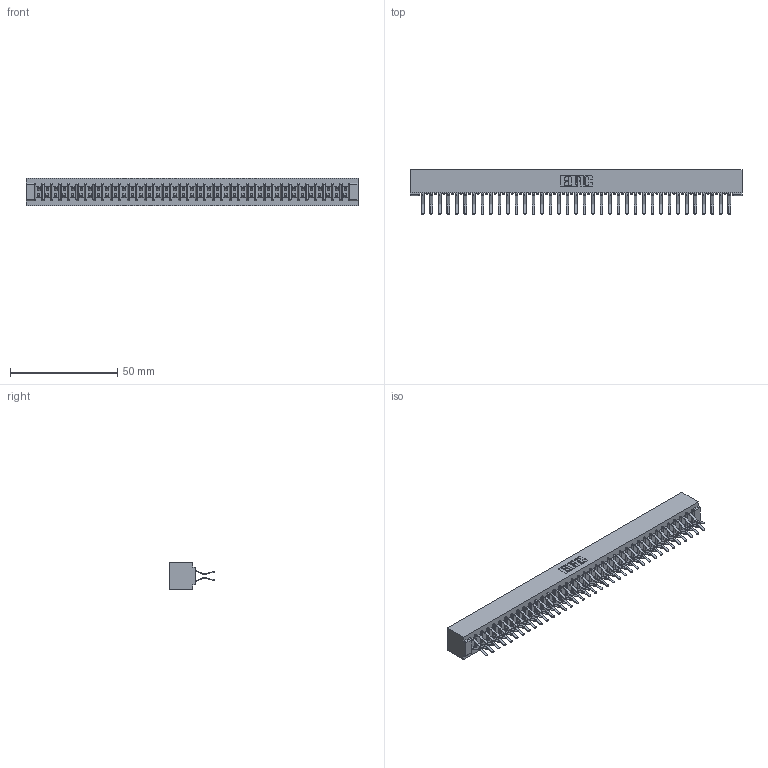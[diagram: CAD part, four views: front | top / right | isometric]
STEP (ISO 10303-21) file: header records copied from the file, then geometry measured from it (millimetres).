
FILE_DESCRIPTION (( 'STEP AP203' ), '1' );
FILE_NAME ('357-074-560-201.STEP', '2018-08-12T21:03:02', ( '' ), ( '' ), 'SwSTEP 2.0', 'SolidWorks 2016', '' );
FILE_SCHEMA (( 'CONFIG_CONTROL_DESIGN' ));
Length unit declared in the file: inch
Products named in the file (3): 307 Part_No Mounting Lugs; 307-290-001_560; 357-074-560-201
Assembly tree (75 placements, depth 2):
  357-074-560-201
    307 Part_No Mounting Lugs
    307-290-001_560  x74
Bounding box: 154.48 x 20.73 x 12.7 mm (x, y, z)
Volume: 17031.8 mm3; surface area: 21549.9 mm2
Topology: 75 solids, 75 shells, 3848 faces, 10807 edges, 7002 vertices
Faces by surface type: plane 2508, cylinder 1264, sphere 76
Entity records: 33346 total; most frequent: CARTESIAN_POINT 5453, ORIENTED_EDGE 5402, DIRECTION 5343, EDGE_CURVE 2701, LINE 2071, VECTOR 2071, VERTEX_POINT 1746, AXIS2_PLACEMENT_3D 1636
